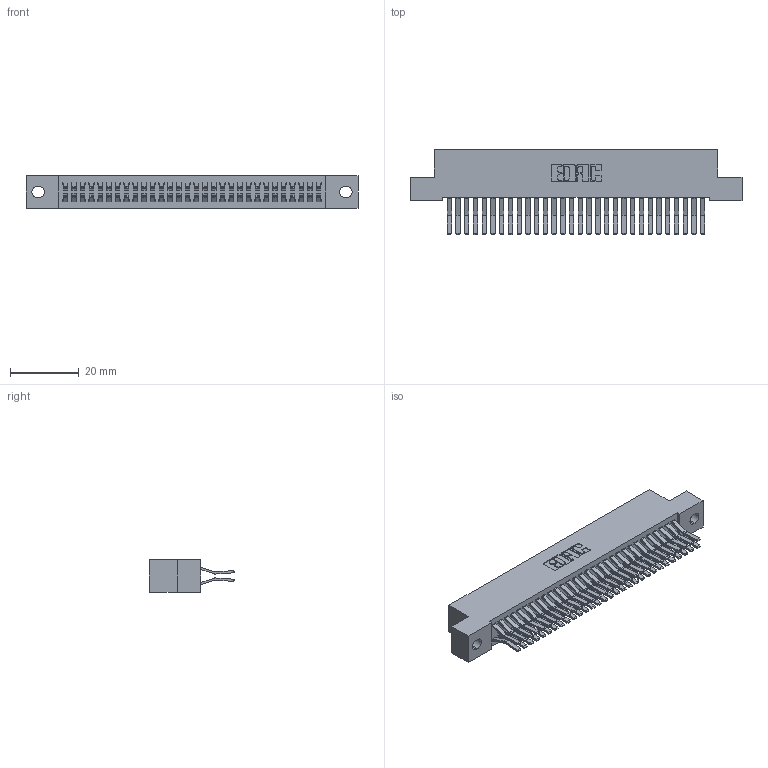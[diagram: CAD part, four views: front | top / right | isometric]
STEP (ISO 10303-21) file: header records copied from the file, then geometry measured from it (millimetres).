
FILE_DESCRIPTION (( 'STEP AP203' ), '1' );
FILE_NAME ('342-060-560-202.STEP', '2019-10-03T13:38:54', ( '' ), ( '' ), 'SwSTEP 2.0', 'SolidWorks 2016', '' );
FILE_SCHEMA (( 'CONFIG_CONTROL_DESIGN' ));
Length unit declared in the file: inch
Products named in the file (3): 342 Part_.128 Slot; 345-292-001_560 Tail; 342-060-560-202
Assembly tree (61 placements, depth 2):
  342-060-560-202
    342 Part_.128 Slot
    345-292-001_560 Tail  x60
Bounding box: 96.52 x 24.78 x 9.4 mm (x, y, z)
Volume: 8957.3 mm3; surface area: 14988.6 mm2
Topology: 61 solids, 61 shells, 3354 faces, 9971 edges, 6566 vertices
Faces by surface type: plane 2230, cylinder 1124
Entity records: 20943 total; most frequent: CARTESIAN_POINT 3486, ORIENTED_EDGE 3422, DIRECTION 3003, EDGE_CURVE 1711, LINE 1579, VECTOR 1579, VERTEX_POINT 1138, AXIS2_PLACEMENT_3D 712
